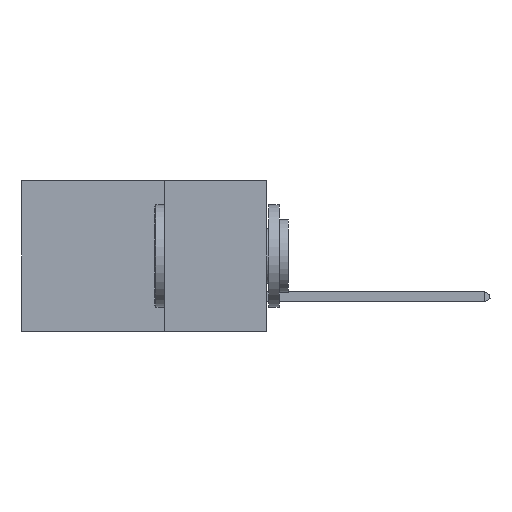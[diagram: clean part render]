
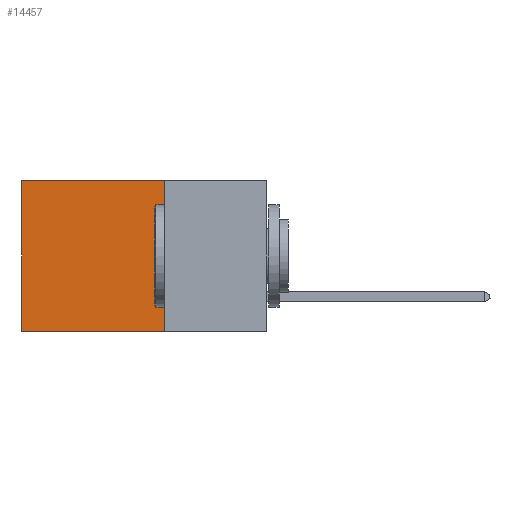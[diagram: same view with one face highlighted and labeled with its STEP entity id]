
A CAD part, left-side view. The second image highlights one B-rep face of the part: STEP entity #14457.
In plain terms, the highlighted planar face has unit normal (-1, 0, 0).
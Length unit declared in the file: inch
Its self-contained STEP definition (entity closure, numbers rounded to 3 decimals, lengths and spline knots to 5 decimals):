
#1545 = EDGE_CURVE ( 'NONE', #14737, #17999, #12228, .T. ) ;
#1969 = CARTESIAN_POINT ( 'NONE',  ( 0.2875, 0.25, 0. ) ) ;
#2365 = VERTEX_POINT ( 'NONE', #11644 ) ;
#2405 = DIRECTION ( 'NONE',  ( 0., 1., 0. ) ) ;
#2747 = VECTOR ( 'NONE', #2405, 39.37008 ) ;
#2905 = CARTESIAN_POINT ( 'NONE',  ( 0.2875, 0.25, -0.37 ) ) ;
#3632 = ORIENTED_EDGE ( 'NONE', *, *, #1545, .F. ) ;
#3978 = DIRECTION ( 'NONE',  ( 0., 0., -1. ) ) ;
#4051 = EDGE_CURVE ( 'NONE', #7286, #2365, #23399, .T. ) ;
#4804 = ORIENTED_EDGE ( 'NONE', *, *, #4051, .T. ) ;
#5758 = EDGE_CURVE ( 'NONE', #2365, #17999, #13436, .T. ) ;
#5854 = AXIS2_PLACEMENT_3D ( 'NONE', #1969, #16065, #3978 ) ;
#7286 = VERTEX_POINT ( 'NONE', #23888 ) ;
#7343 = VECTOR ( 'NONE', #15342, 39.37008 ) ;
#8275 = ORIENTED_EDGE ( 'NONE', *, *, #14603, .F. ) ;
#8417 = CARTESIAN_POINT ( 'NONE',  ( 0.2875, 0.6, 0. ) ) ;
#8726 = VECTOR ( 'NONE', #22469, 39.37008 ) ;
#9945 = LINE ( 'NONE', #22536, #14626 ) ;
#11644 = CARTESIAN_POINT ( 'NONE',  ( 0.2875, 0.6, 0. ) ) ;
#11651 = EDGE_LOOP ( 'NONE', ( #20743, #3632, #8275, #4804 ) ) ;
#12228 = LINE ( 'NONE', #18533, #2747 ) ;
#13323 = CARTESIAN_POINT ( 'NONE',  ( 0.2875, 0.25, 0. ) ) ;
#13436 = LINE ( 'NONE', #8417, #8726 ) ;
#13952 = CARTESIAN_POINT ( 'NONE',  ( 0.2875, 0.6, -0.37 ) ) ;
#14450 = DIRECTION ( 'NONE',  ( 0., 0., -1. ) ) ;
#14457 = ADVANCED_FACE ( 'NONE', ( #23131 ), #24054, .F. ) ;
#14603 = EDGE_CURVE ( 'NONE', #7286, #14737, #9945, .T. ) ;
#14626 = VECTOR ( 'NONE', #14450, 39.37008 ) ;
#14737 = VERTEX_POINT ( 'NONE', #2905 ) ;
#15342 = DIRECTION ( 'NONE',  ( 0., 1., 0. ) ) ;
#16065 = DIRECTION ( 'NONE',  ( 1., 0., 0. ) ) ;
#17999 = VERTEX_POINT ( 'NONE', #13952 ) ;
#18533 = CARTESIAN_POINT ( 'NONE',  ( 0.2875, 0.25, -0.37 ) ) ;
#20743 = ORIENTED_EDGE ( 'NONE', *, *, #5758, .T. ) ;
#22469 = DIRECTION ( 'NONE',  ( 0., 0., -1. ) ) ;
#22536 = CARTESIAN_POINT ( 'NONE',  ( 0.2875, 0.25, 0. ) ) ;
#23131 = FACE_OUTER_BOUND ( 'NONE', #11651, .T. ) ;
#23399 = LINE ( 'NONE', #13323, #7343 ) ;
#23888 = CARTESIAN_POINT ( 'NONE',  ( 0.2875, 0.25, 0. ) ) ;
#24054 = PLANE ( 'NONE',  #5854 ) ;
